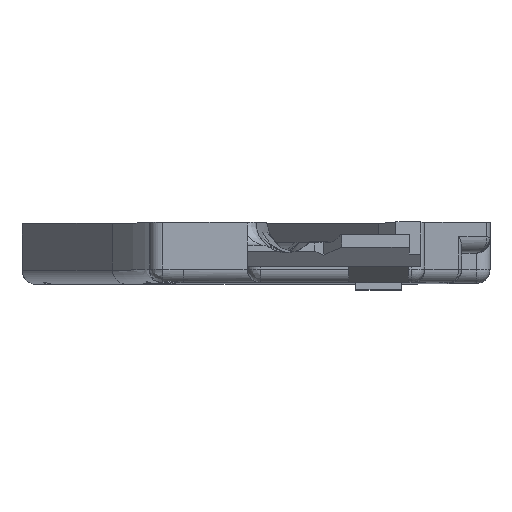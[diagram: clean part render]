
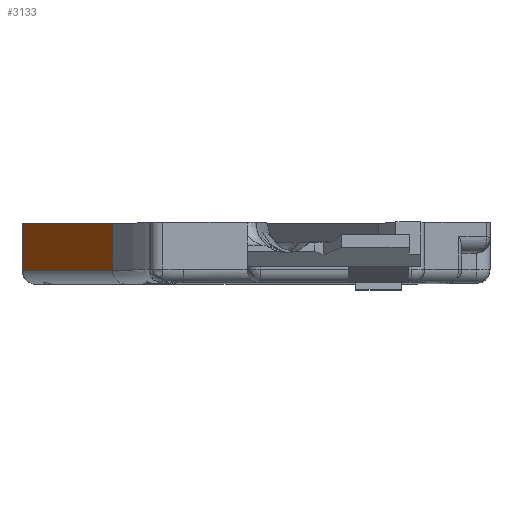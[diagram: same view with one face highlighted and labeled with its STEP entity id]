
A CAD part, top view. The second image highlights one B-rep face of the part: STEP entity #3133.
In plain terms, the highlighted planar face has unit normal (-0.966, 0, 0.259).
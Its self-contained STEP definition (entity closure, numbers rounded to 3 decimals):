
#48=PLANE('',#3391);
#252=FACE_OUTER_BOUND('',#449,.T.);
#449=EDGE_LOOP('',(#2302,#2303,#2304,#2305));
#797=LINE('',#4997,#1013);
#800=LINE('',#5005,#1016);
#801=LINE('',#5007,#1017);
#802=LINE('',#5008,#1018);
#1013=VECTOR('',#3847,10.);
#1016=VECTOR('',#3856,10.);
#1017=VECTOR('',#3857,10.);
#1018=VECTOR('',#3858,10.);
#1378=VERTEX_POINT('',#4990);
#1380=VERTEX_POINT('',#4996);
#1382=VERTEX_POINT('',#5004);
#1383=VERTEX_POINT('',#5006);
#1721=EDGE_CURVE('',#1378,#1380,#797,.T.);
#1725=EDGE_CURVE('',#1382,#1378,#800,.T.);
#1726=EDGE_CURVE('',#1382,#1383,#801,.T.);
#1727=EDGE_CURVE('',#1383,#1380,#802,.T.);
#2302=ORIENTED_EDGE('',*,*,#1721,.F.);
#2303=ORIENTED_EDGE('',*,*,#1725,.F.);
#2304=ORIENTED_EDGE('',*,*,#1726,.T.);
#2305=ORIENTED_EDGE('',*,*,#1727,.T.);
#3133=ADVANCED_FACE('',(#252),#48,.T.);
#3391=AXIS2_PLACEMENT_3D('',#5003,#3854,#3855);
#3847=DIRECTION('',(0.,1.,0.));
#3854=DIRECTION('center_axis',(-0.966,0.,
0.259));
#3855=DIRECTION('ref_axis',(-0.259,0.,-0.966));
#3856=DIRECTION('',(-0.259,0.,-0.966));
#3857=DIRECTION('',(0.,1.,0.));
#3858=DIRECTION('',(-0.259,0.,-0.966));
#4990=CARTESIAN_POINT('',(822.708,-25.378,-145.449));
#4996=CARTESIAN_POINT('',(822.708,-16.727,-145.449));
#4997=CARTESIAN_POINT('',(822.708,-19.477,-145.449));
#5003=CARTESIAN_POINT('Origin',(846.104,-16.727,-58.134));
#5004=CARTESIAN_POINT('',(839.289,-25.378,-83.567));
#5005=CARTESIAN_POINT('',(846.268,-25.378,-57.519));
#5006=CARTESIAN_POINT('',(839.289,-16.727,-83.567));
#5007=CARTESIAN_POINT('',(839.289,-16.727,-83.567));
#5008=CARTESIAN_POINT('',(852.378,-16.727,-34.717));
